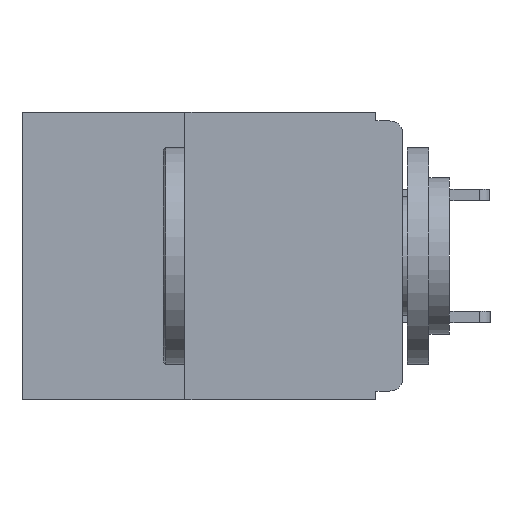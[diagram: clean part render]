
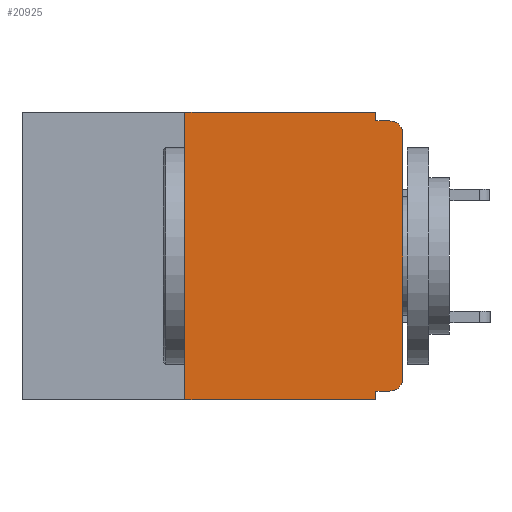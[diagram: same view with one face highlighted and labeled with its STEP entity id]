
A CAD part, left-side view. The second image highlights one B-rep face of the part: STEP entity #20925.
In plain terms, the highlighted planar face has unit normal (-1, 0, 0).
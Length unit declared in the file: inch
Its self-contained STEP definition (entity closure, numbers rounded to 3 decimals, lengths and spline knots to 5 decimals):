
#191 = ORIENTED_EDGE ( 'NONE', *, *, #22139, .F. ) ;
#278 = CARTESIAN_POINT ( 'NONE',  ( 0., 0.015, -0.01 ) ) ;
#296 = ORIENTED_EDGE ( 'NONE', *, *, #13853, .F. ) ;
#474 = ORIENTED_EDGE ( 'NONE', *, *, #18625, .F. ) ;
#519 = VECTOR ( 'NONE', #13983, 39.37008 ) ;
#706 = ORIENTED_EDGE ( 'NONE', *, *, #7624, .T. ) ;
#847 = CARTESIAN_POINT ( 'NONE',  ( 0., 0.031, 0. ) ) ;
#850 = VECTOR ( 'NONE', #6920, 39.37008 ) ;
#1066 = CARTESIAN_POINT ( 'NONE',  ( 0., 0., -0.32 ) ) ;
#1202 = VERTEX_POINT ( 'NONE', #16682 ) ;
#1333 = VERTEX_POINT ( 'NONE', #6176 ) ;
#1368 = DIRECTION ( 'NONE',  ( 0., 1., 0. ) ) ;
#1766 = LINE ( 'NONE', #22260, #11065 ) ;
#1779 = LINE ( 'NONE', #19973, #16597 ) ;
#1815 = DIRECTION ( 'NONE',  ( 0., 0., -1. ) ) ;
#2394 = ORIENTED_EDGE ( 'NONE', *, *, #6578, .F. ) ;
#2681 = ORIENTED_EDGE ( 'NONE', *, *, #6760, .F. ) ;
#2694 = CIRCLE ( 'NONE', #12133, 0.015 ) ;
#2719 = CARTESIAN_POINT ( 'NONE',  ( 0., 0.25, -0.33 ) ) ;
#2822 = VERTEX_POINT ( 'NONE', #7447 ) ;
#2914 = ORIENTED_EDGE ( 'NONE', *, *, #12928, .T. ) ;
#3537 = VECTOR ( 'NONE', #5211, 39.37008 ) ;
#4463 = PLANE ( 'NONE',  #19384 ) ;
#5211 = DIRECTION ( 'NONE',  ( 0., 0., -1. ) ) ;
#5533 = LINE ( 'NONE', #13989, #519 ) ;
#5631 = CARTESIAN_POINT ( 'NONE',  ( 0., 0.031, -0.33 ) ) ;
#5859 = LINE ( 'NONE', #21721, #850 ) ;
#6037 = DIRECTION ( 'NONE',  ( 0., 0., -1. ) ) ;
#6078 = VERTEX_POINT ( 'NONE', #21343 ) ;
#6176 = CARTESIAN_POINT ( 'NONE',  ( 0., 0., -0.305 ) ) ;
#6183 = EDGE_CURVE ( 'NONE', #1333, #6078, #1779, .T. ) ;
#6578 = EDGE_CURVE ( 'NONE', #18745, #2822, #8459, .T. ) ;
#6760 = EDGE_CURVE ( 'NONE', #12588, #18745, #17156, .T. ) ;
#6920 = DIRECTION ( 'NONE',  ( 0., -1., 0. ) ) ;
#6940 = CARTESIAN_POINT ( 'NONE',  ( 0., 0.031, -0.01 ) ) ;
#7447 = CARTESIAN_POINT ( 'NONE',  ( 0., 0.031, -0.33 ) ) ;
#7556 = EDGE_CURVE ( 'NONE', #6078, #20759, #16535, .T. ) ;
#7624 = EDGE_CURVE ( 'NONE', #8114, #2822, #5533, .T. ) ;
#7942 = EDGE_LOOP ( 'NONE', ( #9093, #11050, #15716, #191, #296, #474, #706, #2394, #2681, #2914 ) ) ;
#8114 = VERTEX_POINT ( 'NONE', #8516 ) ;
#8190 = DIRECTION ( 'NONE',  ( 0., 0., -1. ) ) ;
#8459 = LINE ( 'NONE', #5631, #3537 ) ;
#8484 = CARTESIAN_POINT ( 'NONE',  ( 0., 0.031, -0.32 ) ) ;
#8516 = CARTESIAN_POINT ( 'NONE',  ( 0., 0.25, -0.33 ) ) ;
#9093 = ORIENTED_EDGE ( 'NONE', *, *, #6183, .T. ) ;
#10026 = CARTESIAN_POINT ( 'NONE',  ( 0., 0.015, -0.32 ) ) ;
#11050 = ORIENTED_EDGE ( 'NONE', *, *, #7556, .T. ) ;
#11065 = VECTOR ( 'NONE', #22338, 39.37008 ) ;
#11373 = VERTEX_POINT ( 'NONE', #847 ) ;
#11836 = LINE ( 'NONE', #18980, #16743 ) ;
#12133 = AXIS2_PLACEMENT_3D ( 'NONE', #23880, #12987, #1815 ) ;
#12588 = VERTEX_POINT ( 'NONE', #10026 ) ;
#12928 = EDGE_CURVE ( 'NONE', #12588, #1333, #2694, .T. ) ;
#12987 = DIRECTION ( 'NONE',  ( -1., 0., 0. ) ) ;
#13853 = EDGE_CURVE ( 'NONE', #1202, #11373, #5859, .T. ) ;
#13983 = DIRECTION ( 'NONE',  ( 0., -1., 0. ) ) ;
#13989 = CARTESIAN_POINT ( 'NONE',  ( 0., 0.437, -0.33 ) ) ;
#14857 = DIRECTION ( 'NONE',  ( 0., 0., -1. ) ) ;
#14925 = DIRECTION ( 'NONE',  ( -1., 0., 0. ) ) ;
#14931 = CARTESIAN_POINT ( 'NONE',  ( 0., 0.015, -0.025 ) ) ;
#15696 = DIRECTION ( 'NONE',  ( 0., 0., 1. ) ) ;
#15716 = ORIENTED_EDGE ( 'NONE', *, *, #19007, .F. ) ;
#16535 = CIRCLE ( 'NONE', #20173, 0.015 ) ;
#16597 = VECTOR ( 'NONE', #16750, 39.37008 ) ;
#16682 = CARTESIAN_POINT ( 'NONE',  ( 0., 0.25, 0. ) ) ;
#16743 = VECTOR ( 'NONE', #6037, 39.37008 ) ;
#16750 = DIRECTION ( 'NONE',  ( 0., 0., 1. ) ) ;
#17156 = LINE ( 'NONE', #1066, #19176 ) ;
#17193 = VECTOR ( 'NONE', #15696, 39.37008 ) ;
#17411 = CARTESIAN_POINT ( 'NONE',  ( 0., 0.437, 0. ) ) ;
#18625 = EDGE_CURVE ( 'NONE', #8114, #1202, #20952, .T. ) ;
#18745 = VERTEX_POINT ( 'NONE', #8484 ) ;
#18797 = VERTEX_POINT ( 'NONE', #6940 ) ;
#18980 = CARTESIAN_POINT ( 'NONE',  ( 0., 0.031, 0. ) ) ;
#19007 = EDGE_CURVE ( 'NONE', #18797, #20759, #1766, .T. ) ;
#19090 = FACE_OUTER_BOUND ( 'NONE', #7942, .T. ) ;
#19176 = VECTOR ( 'NONE', #1368, 39.37008 ) ;
#19285 = DIRECTION ( 'NONE',  ( 1., 0., 0. ) ) ;
#19384 = AXIS2_PLACEMENT_3D ( 'NONE', #17411, #19285, #8190 ) ;
#19973 = CARTESIAN_POINT ( 'NONE',  ( 0., 0., 0. ) ) ;
#20173 = AXIS2_PLACEMENT_3D ( 'NONE', #14931, #14925, #14857 ) ;
#20759 = VERTEX_POINT ( 'NONE', #278 ) ;
#20925 = ADVANCED_FACE ( 'NONE', ( #19090 ), #4463, .F. ) ;
#20952 = LINE ( 'NONE', #2719, #17193 ) ;
#21343 = CARTESIAN_POINT ( 'NONE',  ( 0., 0., -0.025 ) ) ;
#21721 = CARTESIAN_POINT ( 'NONE',  ( 0., 0.437, 0. ) ) ;
#22139 = EDGE_CURVE ( 'NONE', #11373, #18797, #11836, .T. ) ;
#22260 = CARTESIAN_POINT ( 'NONE',  ( 0., 0., -0.01 ) ) ;
#22338 = DIRECTION ( 'NONE',  ( 0., -1., 0. ) ) ;
#23880 = CARTESIAN_POINT ( 'NONE',  ( 0., 0.015, -0.305 ) ) ;
